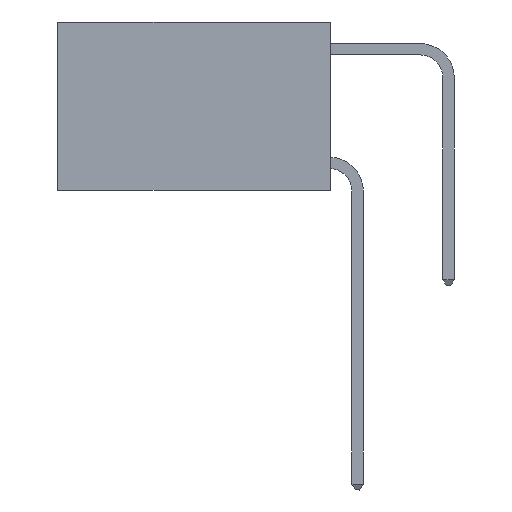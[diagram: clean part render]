
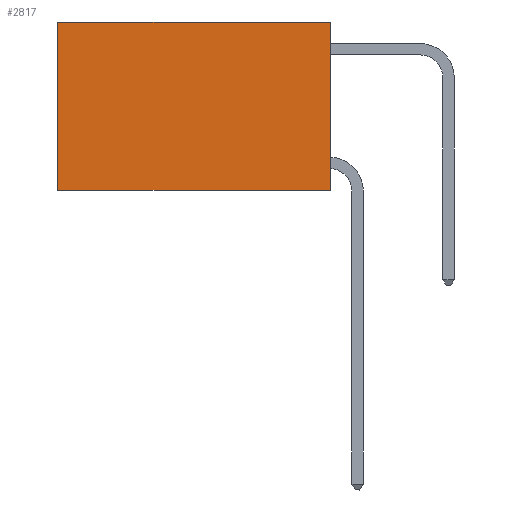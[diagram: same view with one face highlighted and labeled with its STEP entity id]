
A CAD part, left-side view. The second image highlights one B-rep face of the part: STEP entity #2817.
In plain terms, the highlighted planar face has unit normal (-1, 0, 0).
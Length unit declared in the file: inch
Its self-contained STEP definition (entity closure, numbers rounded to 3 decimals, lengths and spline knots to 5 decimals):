
#423 = LINE ( 'NONE', #7361, #4073 ) ;
#981 = CARTESIAN_POINT ( 'NONE',  ( 0.2625, 0., 0. ) ) ;
#1055 = CARTESIAN_POINT ( 'NONE',  ( 0.2625, 0.6, 0. ) ) ;
#2609 = ORIENTED_EDGE ( 'NONE', *, *, #3169, .T. ) ;
#2739 = CARTESIAN_POINT ( 'NONE',  ( 0.2625, 0.6, 0. ) ) ;
#2817 = ADVANCED_FACE ( 'NONE', ( #8619 ), #7928, .F. ) ;
#2825 = EDGE_CURVE ( 'NONE', #15501, #11832, #8200, .T. ) ;
#2954 = EDGE_CURVE ( 'NONE', #10413, #11832, #17212, .T. ) ;
#2962 = DIRECTION ( 'NONE',  ( 0., 0., -1. ) ) ;
#3169 = EDGE_CURVE ( 'NONE', #7184, #10413, #10736, .T. ) ;
#3229 = ORIENTED_EDGE ( 'NONE', *, *, #2825, .F. ) ;
#3468 = VECTOR ( 'NONE', #16158, 39.37008 ) ;
#3794 = AXIS2_PLACEMENT_3D ( 'NONE', #7836, #7575, #7549 ) ;
#3929 = CARTESIAN_POINT ( 'NONE',  ( 0.2625, 0.6, -0.37 ) ) ;
#4073 = VECTOR ( 'NONE', #15482, 39.37008 ) ;
#4431 = CARTESIAN_POINT ( 'NONE',  ( 0.2625, 0., -0.37 ) ) ;
#4542 = VECTOR ( 'NONE', #7485, 39.37008 ) ;
#7184 = VERTEX_POINT ( 'NONE', #981 ) ;
#7340 = CARTESIAN_POINT ( 'NONE',  ( 0.2625, 0., -0.37 ) ) ;
#7361 = CARTESIAN_POINT ( 'NONE',  ( 0.2625, 0., 0. ) ) ;
#7485 = DIRECTION ( 'NONE',  ( 0., 1., 0. ) ) ;
#7549 = DIRECTION ( 'NONE',  ( 0., 0., -1. ) ) ;
#7575 = DIRECTION ( 'NONE',  ( 1., 0., 0. ) ) ;
#7591 = EDGE_CURVE ( 'NONE', #7184, #15501, #423, .T. ) ;
#7836 = CARTESIAN_POINT ( 'NONE',  ( 0.2625, 0., 0. ) ) ;
#7928 = PLANE ( 'NONE',  #3794 ) ;
#8200 = LINE ( 'NONE', #7340, #4542 ) ;
#8619 = FACE_OUTER_BOUND ( 'NONE', #13124, .T. ) ;
#9070 = ORIENTED_EDGE ( 'NONE', *, *, #7591, .F. ) ;
#10413 = VERTEX_POINT ( 'NONE', #1055 ) ;
#10736 = LINE ( 'NONE', #13625, #3468 ) ;
#11832 = VERTEX_POINT ( 'NONE', #3929 ) ;
#13124 = EDGE_LOOP ( 'NONE', ( #17100, #3229, #9070, #2609 ) ) ;
#13625 = CARTESIAN_POINT ( 'NONE',  ( 0.2625, 0., 0. ) ) ;
#13725 = VECTOR ( 'NONE', #2962, 39.37008 ) ;
#15482 = DIRECTION ( 'NONE',  ( 0., 0., -1. ) ) ;
#15501 = VERTEX_POINT ( 'NONE', #4431 ) ;
#16158 = DIRECTION ( 'NONE',  ( 0., 1., 0. ) ) ;
#17100 = ORIENTED_EDGE ( 'NONE', *, *, #2954, .T. ) ;
#17212 = LINE ( 'NONE', #2739, #13725 ) ;
